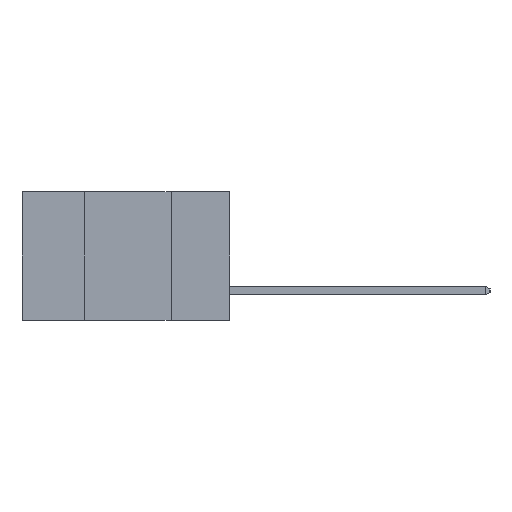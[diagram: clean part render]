
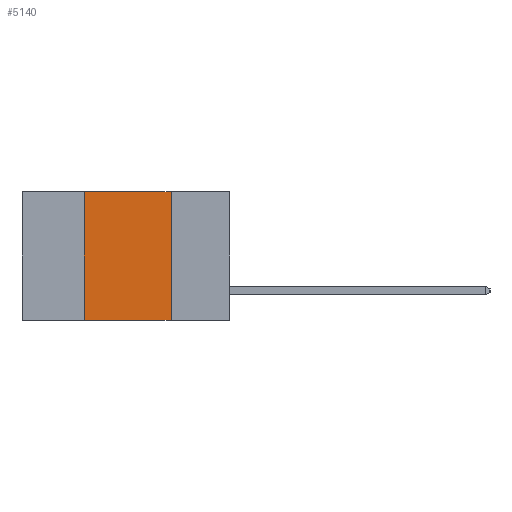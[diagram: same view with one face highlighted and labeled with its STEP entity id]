
A CAD part, left-side view. The second image highlights one B-rep face of the part: STEP entity #5140.
In plain terms, the highlighted planar face has unit normal (-1, 0, 0).
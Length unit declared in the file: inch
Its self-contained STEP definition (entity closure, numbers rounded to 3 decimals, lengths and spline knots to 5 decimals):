
#54 = VERTEX_POINT ( 'NONE', #436 ) ;
#182 = VERTEX_POINT ( 'NONE', #1407 ) ;
#436 = CARTESIAN_POINT ( 'NONE',  ( 0., 0.42, -0.37 ) ) ;
#439 = CARTESIAN_POINT ( 'NONE',  ( 0., 0.6, -0.37 ) ) ;
#1305 = VERTEX_POINT ( 'NONE', #2834 ) ;
#1407 = CARTESIAN_POINT ( 'NONE',  ( 0., 0.17, -0.37 ) ) ;
#1510 = LINE ( 'NONE', #3787, #3616 ) ;
#1684 = EDGE_LOOP ( 'NONE', ( #2742, #2866, #5124, #3125 ) ) ;
#1811 = LINE ( 'NONE', #10196, #8126 ) ;
#1940 = CARTESIAN_POINT ( 'NONE',  ( 0., 0.17, 0. ) ) ;
#2383 = VECTOR ( 'NONE', #3097, 39.37008 ) ;
#2742 = ORIENTED_EDGE ( 'NONE', *, *, #9709, .F. ) ;
#2834 = CARTESIAN_POINT ( 'NONE',  ( 0., 0.42, 0. ) ) ;
#2866 = ORIENTED_EDGE ( 'NONE', *, *, #10091, .F. ) ;
#3097 = DIRECTION ( 'NONE',  ( 0., -1., 0. ) ) ;
#3125 = ORIENTED_EDGE ( 'NONE', *, *, #9645, .T. ) ;
#3616 = VECTOR ( 'NONE', #9243, 39.37008 ) ;
#3784 = DIRECTION ( 'NONE',  ( 1., 0., 0. ) ) ;
#3787 = CARTESIAN_POINT ( 'NONE',  ( 0., 0.6, 0. ) ) ;
#5124 = ORIENTED_EDGE ( 'NONE', *, *, #7729, .F. ) ;
#5140 = ADVANCED_FACE ( 'NONE', ( #6210 ), #8516, .F. ) ;
#5730 = DIRECTION ( 'NONE',  ( 0., 0., -1. ) ) ;
#6210 = FACE_OUTER_BOUND ( 'NONE', #1684, .T. ) ;
#6293 = CARTESIAN_POINT ( 'NONE',  ( 0., 0.6, 0. ) ) ;
#6891 = LINE ( 'NONE', #439, #2383 ) ;
#7729 = EDGE_CURVE ( 'NONE', #54, #1305, #8432, .T. ) ;
#8126 = VECTOR ( 'NONE', #5730, 39.37008 ) ;
#8196 = VECTOR ( 'NONE', #8716, 39.37008 ) ;
#8432 = LINE ( 'NONE', #9419, #8196 ) ;
#8516 = PLANE ( 'NONE',  #8701 ) ;
#8701 = AXIS2_PLACEMENT_3D ( 'NONE', #6293, #3784, #9208 ) ;
#8716 = DIRECTION ( 'NONE',  ( 0., 0., 1. ) ) ;
#9208 = DIRECTION ( 'NONE',  ( 0., 0., -1. ) ) ;
#9243 = DIRECTION ( 'NONE',  ( 0., -1., 0. ) ) ;
#9419 = CARTESIAN_POINT ( 'NONE',  ( 0., 0.42, 0. ) ) ;
#9426 = VERTEX_POINT ( 'NONE', #1940 ) ;
#9645 = EDGE_CURVE ( 'NONE', #54, #182, #6891, .T. ) ;
#9709 = EDGE_CURVE ( 'NONE', #9426, #182, #1811, .T. ) ;
#10091 = EDGE_CURVE ( 'NONE', #1305, #9426, #1510, .T. ) ;
#10196 = CARTESIAN_POINT ( 'NONE',  ( 0., 0.17, 0. ) ) ;
